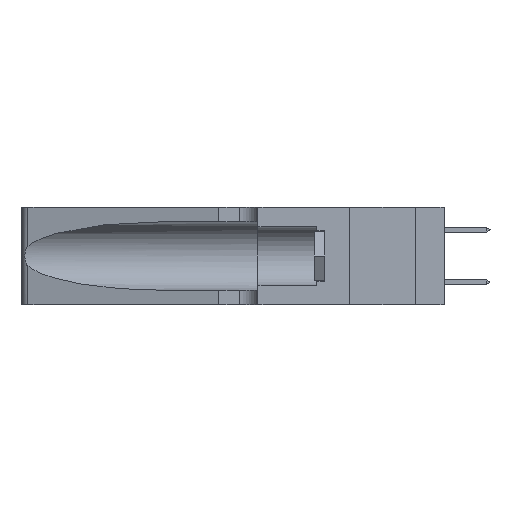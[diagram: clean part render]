
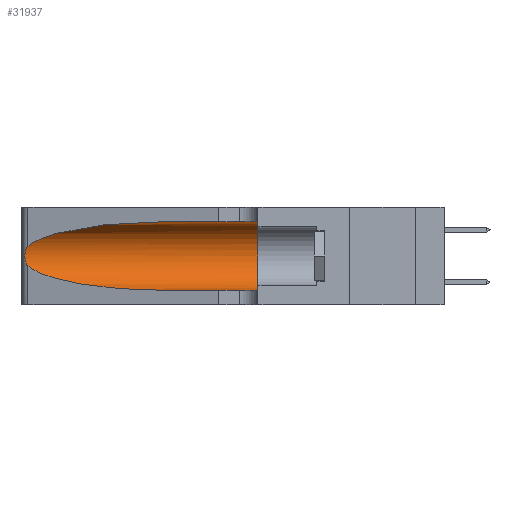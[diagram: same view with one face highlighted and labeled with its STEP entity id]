
A CAD part, left-side view. The second image highlights one B-rep face of the part: STEP entity #31937.
In plain terms, the highlighted cylindrical face has radius 3.308 mm (diameter 6.617 mm), a partial arc.
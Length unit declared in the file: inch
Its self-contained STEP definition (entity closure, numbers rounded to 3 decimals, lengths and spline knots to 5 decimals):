
#303 = CARTESIAN_POINT ( 'NONE',  ( 0.25555, 1.22993, 0.14849 ) ) ;
#355 = EDGE_LOOP ( 'NONE', ( #5012, #7694, #1753, #17218, #4623, #4968 ) ) ;
#360 = CARTESIAN_POINT ( 'NONE',  ( 0.25487, 1.22718, 0.14631 ) ) ;
#391 = VERTEX_POINT ( 'NONE', #599 ) ;
#463 = CARTESIAN_POINT ( 'NONE',  ( 0.25487, 1.22718, 0.14631 ) ) ;
#599 = CARTESIAN_POINT ( 'NONE',  ( 0.25487, 1.22718, 0.22369 ) ) ;
#1640 = LINE ( 'NONE', #19209, #22182 ) ;
#1753 = ORIENTED_EDGE ( 'NONE', *, *, #29704, .T. ) ;
#2884 = CARTESIAN_POINT ( 'NONE',  ( 0.2373, 1.15595, 0.08982 ) ) ;
#3043 = EDGE_CURVE ( 'NONE', #3068, #27627, #1640, .T. ) ;
#3068 = VERTEX_POINT ( 'NONE', #6872 ) ;
#3309 = CARTESIAN_POINT ( 'NONE',  ( 0.18966, 0.96281, 0.31525 ) ) ;
#3458 = LINE ( 'NONE', #25620, #27552 ) ;
#3482 = DIRECTION ( 'NONE',  ( 0., -1., 0. ) ) ;
#3498 = CARTESIAN_POINT ( 'NONE',  ( 0.26018, 1.23835, 0.19895 ) ) ;
#3632 = CARTESIAN_POINT ( 'NONE',  ( 0.25487, 1.22718, 0.22369 ) ) ;
#4623 = ORIENTED_EDGE ( 'NONE', *, *, #26709, .F. ) ;
#4717 = CARTESIAN_POINT ( 'NONE',  ( 0.1305, 0.35, 0.31525 ) ) ;
#4968 = ORIENTED_EDGE ( 'NONE', *, *, #3043, .F. ) ;
#5012 = ORIENTED_EDGE ( 'NONE', *, *, #5118, .T. ) ;
#5118 = EDGE_CURVE ( 'NONE', #3068, #391, #7438, .T. ) ;
#5612 = CARTESIAN_POINT ( 'NONE',  ( 0.18966, 0.96281, 0.05475 ) ) ;
#6872 = CARTESIAN_POINT ( 'NONE',  ( 0.1305, 0.72297, 0.31525 ) ) ;
#7438 =( BOUNDED_CURVE ( )  B_SPLINE_CURVE ( 3, ( #13047, #3309, #11121, #3632 ),
 .UNSPECIFIED., .F., .T. ) 
 B_SPLINE_CURVE_WITH_KNOTS ( ( 4, 4 ),
 ( 1.5708, 2.84003 ),
 .UNSPECIFIED. ) 
 CURVE ( )  GEOMETRIC_REPRESENTATION_ITEM ( )  RATIONAL_B_SPLINE_CURVE ( ( 1., 0.87, 0.87, 1. ) ) 
 REPRESENTATION_ITEM ( '' )  );
#7694 = ORIENTED_EDGE ( 'NONE', *, *, #20813, .T. ) ;
#8772 = DIRECTION ( 'NONE',  ( 0., 0., 1. ) ) ;
#9243 = CARTESIAN_POINT ( 'NONE',  ( 0.1305, 1.61858, 0.185 ) ) ;
#9421 = CIRCLE ( 'NONE', #21971, 0.13025 ) ;
#9815 = VERTEX_POINT ( 'NONE', #13976 ) ;
#11121 = CARTESIAN_POINT ( 'NONE',  ( 0.2373, 1.15595, 0.28018 ) ) ;
#11732 = DIRECTION ( 'NONE',  ( 0., -1., 0. ) ) ;
#12130 = CYLINDRICAL_SURFACE ( 'NONE', #14200, 0.13025 ) ;
#12276 = EDGE_CURVE ( 'NONE', #19179, #9815, #3458, .T. ) ;
#13047 = CARTESIAN_POINT ( 'NONE',  ( 0.1305, 0.72297, 0.31525 ) ) ;
#13582 = CARTESIAN_POINT ( 'NONE',  ( 0.25856, 1.23593, 0.16098 ) ) ;
#13976 = CARTESIAN_POINT ( 'NONE',  ( 0.1305, 0.35, 0.05475 ) ) ;
#14200 = AXIS2_PLACEMENT_3D ( 'NONE', #9243, #11732, #31680 ) ;
#15478 = DIRECTION ( 'NONE',  ( 0., 1., 0. ) ) ;
#16666 = CARTESIAN_POINT ( 'NONE',  ( 0.25787, 1.23484, 0.2124 ) ) ;
#17218 = ORIENTED_EDGE ( 'NONE', *, *, #12276, .T. ) ;
#18322 =( BOUNDED_CURVE ( )  B_SPLINE_CURVE ( 3, ( #360, #2884, #5612, #20544 ),
 .UNSPECIFIED., .F., .F. ) 
 B_SPLINE_CURVE_WITH_KNOTS ( ( 4, 4 ),
 ( 3.44316, 4.71239 ),
 .UNSPECIFIED. ) 
 CURVE ( )  GEOMETRIC_REPRESENTATION_ITEM ( )  RATIONAL_B_SPLINE_CURVE ( ( 1., 0.87, 0.87, 1. ) ) 
 REPRESENTATION_ITEM ( '' )  );
#19176 = DIRECTION ( 'NONE',  ( 0., -1., 0. ) ) ;
#19179 = VERTEX_POINT ( 'NONE', #23222 ) ;
#19209 = CARTESIAN_POINT ( 'NONE',  ( 0.1305, 1.61858, 0.31525 ) ) ;
#19805 = CARTESIAN_POINT ( 'NONE',  ( 0.25854, 1.2359, 0.20912 ) ) ;
#20544 = CARTESIAN_POINT ( 'NONE',  ( 0.1305, 0.72297, 0.05475 ) ) ;
#20813 = EDGE_CURVE ( 'NONE', #391, #26428, #21739, .T. ) ;
#21739 = B_SPLINE_CURVE_WITH_KNOTS ( 'NONE', 3,
 ( #29906, #29710, #22062, #16666, #19805, #3498, #28162, #22998, #28387, #13582, #23095, #21940, #303, #28688 ),
 .UNSPECIFIED., .F., .F.,
 ( 4, 2, 2, 2, 2, 2, 4 ),
 ( 0., 0.00027, 0.00053, 0.00107, 0.0016, 0.00187, 0.00214 ),
 .UNSPECIFIED. ) ;
#21940 = CARTESIAN_POINT ( 'NONE',  ( 0.25639, 1.23186, 0.15144 ) ) ;
#21971 = AXIS2_PLACEMENT_3D ( 'NONE', #30352, #15478, #8772 ) ;
#22062 = CARTESIAN_POINT ( 'NONE',  ( 0.25639, 1.23184, 0.21858 ) ) ;
#22182 = VECTOR ( 'NONE', #19176, 39.37008 ) ;
#22998 = CARTESIAN_POINT ( 'NONE',  ( 0.26075, 1.23896, 0.178 ) ) ;
#23095 = CARTESIAN_POINT ( 'NONE',  ( 0.25789, 1.23486, 0.15765 ) ) ;
#23222 = CARTESIAN_POINT ( 'NONE',  ( 0.1305, 0.72297, 0.05475 ) ) ;
#24560 = FACE_OUTER_BOUND ( 'NONE', #355, .T. ) ;
#25620 = CARTESIAN_POINT ( 'NONE',  ( 0.1305, 1.61858, 0.05475 ) ) ;
#26428 = VERTEX_POINT ( 'NONE', #463 ) ;
#26709 = EDGE_CURVE ( 'NONE', #27627, #9815, #9421, .T. ) ;
#27552 = VECTOR ( 'NONE', #3482, 39.37008 ) ;
#27627 = VERTEX_POINT ( 'NONE', #4717 ) ;
#28162 = CARTESIAN_POINT ( 'NONE',  ( 0.26075, 1.23896, 0.19203 ) ) ;
#28387 = CARTESIAN_POINT ( 'NONE',  ( 0.26017, 1.23833, 0.17102 ) ) ;
#28688 = CARTESIAN_POINT ( 'NONE',  ( 0.25487, 1.22718, 0.14631 ) ) ;
#29704 = EDGE_CURVE ( 'NONE', #26428, #19179, #18322, .T. ) ;
#29710 = CARTESIAN_POINT ( 'NONE',  ( 0.25555, 1.22994, 0.2215 ) ) ;
#29906 = CARTESIAN_POINT ( 'NONE',  ( 0.25487, 1.22718, 0.22369 ) ) ;
#30352 = CARTESIAN_POINT ( 'NONE',  ( 0.1305, 0.35, 0.185 ) ) ;
#31680 = DIRECTION ( 'NONE',  ( 0., 0., -1. ) ) ;
#31937 = ADVANCED_FACE ( 'NONE', ( #24560 ), #12130, .F. ) ;
